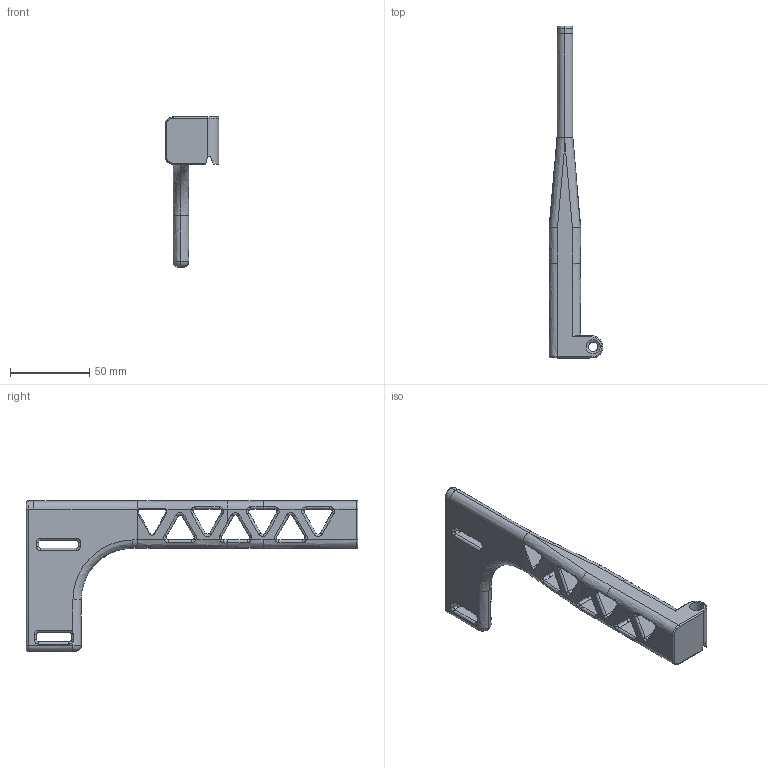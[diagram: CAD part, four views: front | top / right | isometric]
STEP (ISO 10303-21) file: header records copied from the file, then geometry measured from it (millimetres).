
FILE_DESCRIPTION(/* description */ (''),/* implementation_level */ '2;1');
FILE_NAME(/* name */ 'Brace Arm.step',/* time_stamp */ '2021-01-18T14:21:56-07:00',/* author */ (''),/* organization */ (''),/* preprocessor_version */ 'ST-DEVELOPER v18.1',/* originating_system */ 'Autodesk Translation Framework v9.7.1.1290',/* authorisation */ '');
FILE_SCHEMA (('AUTOMOTIVE_DESIGN { 1 0 10303 214 3 1 1 }'));
Length unit declared in the file: inch
Products named in the file (1): Space Gun Beta Ready
Bounding box: 34 x 210 x 95 mm (x, y, z)
Volume: 95902 mm3; surface area: 29849.7 mm2
Topology: 1 solids, 1 shells, 308 faces, 787 edges, 464 vertices
Faces by surface type: bspline 243, plane 48, cylinder 14, torus 2, cone 1
Full cylindrical faces by diameter (mm): 6 x1, 9 x1
Entity records: 19354 total; most frequent: CARTESIAN_POINT 14014, ORIENTED_EDGE 1574, EDGE_CURVE 787, B_SPLINE_CURVE_WITH_KNOTS 695, VERTEX_POINT 464, EDGE_LOOP 311, FACE_OUTER_BOUND 308, ADVANCED_FACE 308
